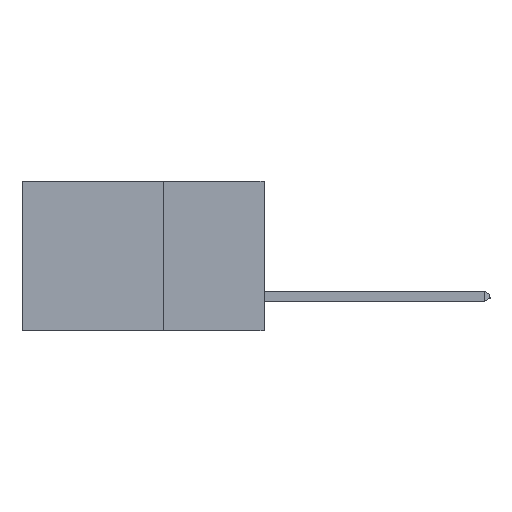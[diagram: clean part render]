
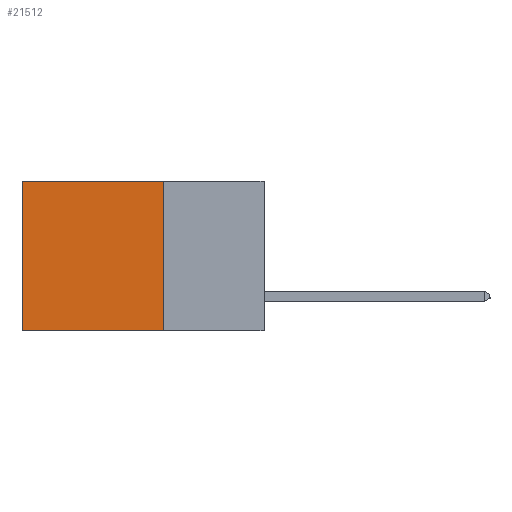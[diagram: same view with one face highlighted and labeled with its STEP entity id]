
A CAD part, left-side view. The second image highlights one B-rep face of the part: STEP entity #21512.
In plain terms, the highlighted planar face has unit normal (-1, 0, 0).
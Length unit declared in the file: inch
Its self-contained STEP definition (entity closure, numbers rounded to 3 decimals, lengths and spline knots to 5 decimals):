
#491 = ORIENTED_EDGE ( 'NONE', *, *, #26133, .F. ) ;
#1267 = LINE ( 'NONE', #6630, #24991 ) ;
#1628 = DIRECTION ( 'NONE',  ( 0., 1., 0. ) ) ;
#2511 = CARTESIAN_POINT ( 'NONE',  ( 0.298, 0.25, 0. ) ) ;
#2514 = DIRECTION ( 'NONE',  ( 1., 0., 0. ) ) ;
#5749 = CARTESIAN_POINT ( 'NONE',  ( 0.298, 0.25, -0.37 ) ) ;
#5871 = VERTEX_POINT ( 'NONE', #23422 ) ;
#6426 = EDGE_CURVE ( 'NONE', #10935, #9215, #25578, .T. ) ;
#6630 = CARTESIAN_POINT ( 'NONE',  ( 0.298, 0.6, 0. ) ) ;
#8756 = CARTESIAN_POINT ( 'NONE',  ( 0.298, 0.25, 0. ) ) ;
#9215 = VERTEX_POINT ( 'NONE', #12763 ) ;
#10935 = VERTEX_POINT ( 'NONE', #22626 ) ;
#12763 = CARTESIAN_POINT ( 'NONE',  ( 0.298, 0.6, 0. ) ) ;
#12857 = VECTOR ( 'NONE', #16185, 39.37008 ) ;
#13216 = EDGE_CURVE ( 'NONE', #9215, #5871, #1267, .T. ) ;
#14535 = LINE ( 'NONE', #2511, #20039 ) ;
#14536 = EDGE_CURVE ( 'NONE', #19755, #5871, #18400, .T. ) ;
#15890 = ORIENTED_EDGE ( 'NONE', *, *, #13216, .T. ) ;
#16185 = DIRECTION ( 'NONE',  ( 0., 1., 0. ) ) ;
#17899 = ORIENTED_EDGE ( 'NONE', *, *, #6426, .T. ) ;
#18400 = LINE ( 'NONE', #27688, #12857 ) ;
#19066 = CARTESIAN_POINT ( 'NONE',  ( 0.298, 0.25, 0. ) ) ;
#19170 = DIRECTION ( 'NONE',  ( 0., 0., -1. ) ) ;
#19363 = VECTOR ( 'NONE', #1628, 39.37008 ) ;
#19755 = VERTEX_POINT ( 'NONE', #5749 ) ;
#20039 = VECTOR ( 'NONE', #28530, 39.37008 ) ;
#20854 = DIRECTION ( 'NONE',  ( 0., 0., -1. ) ) ;
#21512 = ADVANCED_FACE ( 'NONE', ( #29269 ), #28434, .F. ) ;
#22626 = CARTESIAN_POINT ( 'NONE',  ( 0.298, 0.25, 0. ) ) ;
#23422 = CARTESIAN_POINT ( 'NONE',  ( 0.298, 0.6, -0.37 ) ) ;
#23535 = EDGE_LOOP ( 'NONE', ( #15890, #25582, #491, #17899 ) ) ;
#24991 = VECTOR ( 'NONE', #20854, 39.37008 ) ;
#25578 = LINE ( 'NONE', #8756, #19363 ) ;
#25582 = ORIENTED_EDGE ( 'NONE', *, *, #14536, .F. ) ;
#26133 = EDGE_CURVE ( 'NONE', #10935, #19755, #14535, .T. ) ;
#27688 = CARTESIAN_POINT ( 'NONE',  ( 0.298, 0.25, -0.37 ) ) ;
#28434 = PLANE ( 'NONE',  #30355 ) ;
#28530 = DIRECTION ( 'NONE',  ( 0., 0., -1. ) ) ;
#29269 = FACE_OUTER_BOUND ( 'NONE', #23535, .T. ) ;
#30355 = AXIS2_PLACEMENT_3D ( 'NONE', #19066, #2514, #19170 ) ;
